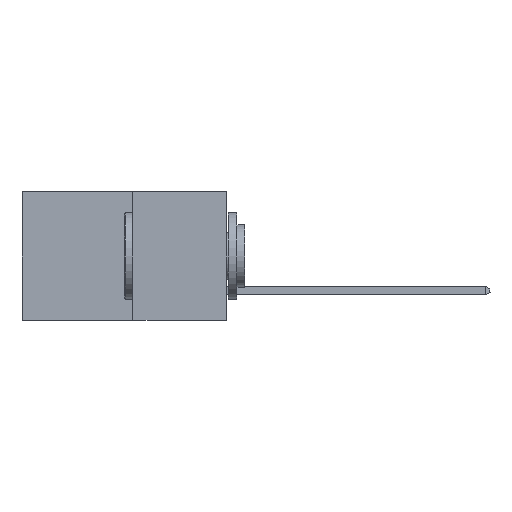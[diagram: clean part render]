
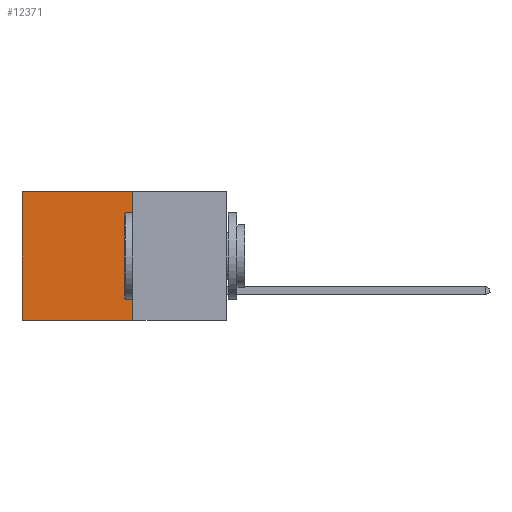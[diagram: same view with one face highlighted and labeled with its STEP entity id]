
A CAD part, left-side view. The second image highlights one B-rep face of the part: STEP entity #12371.
In plain terms, the highlighted planar face has unit normal (-1, 0, 0).
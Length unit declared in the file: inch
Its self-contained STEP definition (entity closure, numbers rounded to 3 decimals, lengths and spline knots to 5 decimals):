
#427 = VERTEX_POINT ( 'NONE', #11050 ) ;
#567 = LINE ( 'NONE', #4258, #4537 ) ;
#1040 = EDGE_CURVE ( 'NONE', #4938, #16372, #567, .T. ) ;
#2025 = ORIENTED_EDGE ( 'NONE', *, *, #11474, .F. ) ;
#2215 = CARTESIAN_POINT ( 'NONE',  ( 0.277, 0.27, -0.37 ) ) ;
#3287 = DIRECTION ( 'NONE',  ( 1., 0., 0. ) ) ;
#3907 = CARTESIAN_POINT ( 'NONE',  ( 0.277, 0.59, -0.37 ) ) ;
#4258 = CARTESIAN_POINT ( 'NONE',  ( 0.277, 0.27, -0.37 ) ) ;
#4537 = VECTOR ( 'NONE', #16765, 39.37008 ) ;
#4938 = VERTEX_POINT ( 'NONE', #2215 ) ;
#5382 = DIRECTION ( 'NONE',  ( 0., 1., 0. ) ) ;
#5526 = CARTESIAN_POINT ( 'NONE',  ( 0.277, 0.27, 0. ) ) ;
#5700 = CARTESIAN_POINT ( 'NONE',  ( 0.277, 0.27, 0. ) ) ;
#5919 = AXIS2_PLACEMENT_3D ( 'NONE', #13514, #3287, #15207 ) ;
#6497 = VERTEX_POINT ( 'NONE', #5700 ) ;
#7149 = EDGE_CURVE ( 'NONE', #6497, #427, #11401, .T. ) ;
#7910 = EDGE_LOOP ( 'NONE', ( #12688, #13218, #2025, #17721 ) ) ;
#8365 = PLANE ( 'NONE',  #5919 ) ;
#9088 = LINE ( 'NONE', #21373, #17076 ) ;
#9646 = CARTESIAN_POINT ( 'NONE',  ( 0.277, 0.59, -0.37 ) ) ;
#10531 = LINE ( 'NONE', #3907, #18984 ) ;
#11050 = CARTESIAN_POINT ( 'NONE',  ( 0.277, 0.59, 0. ) ) ;
#11401 = LINE ( 'NONE', #5526, #19810 ) ;
#11474 = EDGE_CURVE ( 'NONE', #6497, #4938, #9088, .T. ) ;
#12304 = FACE_OUTER_BOUND ( 'NONE', #7910, .T. ) ;
#12371 = ADVANCED_FACE ( 'NONE', ( #12304 ), #8365, .F. ) ;
#12688 = ORIENTED_EDGE ( 'NONE', *, *, #15524, .T. ) ;
#13218 = ORIENTED_EDGE ( 'NONE', *, *, #1040, .F. ) ;
#13514 = CARTESIAN_POINT ( 'NONE',  ( 0.277, 0.27, -0.37 ) ) ;
#14130 = DIRECTION ( 'NONE',  ( 0., 0., -1. ) ) ;
#15207 = DIRECTION ( 'NONE',  ( 0., 0., -1. ) ) ;
#15524 = EDGE_CURVE ( 'NONE', #427, #16372, #10531, .T. ) ;
#16372 = VERTEX_POINT ( 'NONE', #9646 ) ;
#16765 = DIRECTION ( 'NONE',  ( 0., 1., 0. ) ) ;
#17076 = VECTOR ( 'NONE', #18046, 39.37008 ) ;
#17721 = ORIENTED_EDGE ( 'NONE', *, *, #7149, .T. ) ;
#18046 = DIRECTION ( 'NONE',  ( 0., 0., -1. ) ) ;
#18984 = VECTOR ( 'NONE', #14130, 39.37008 ) ;
#19810 = VECTOR ( 'NONE', #5382, 39.37008 ) ;
#21373 = CARTESIAN_POINT ( 'NONE',  ( 0.277, 0.27, -0.37 ) ) ;
